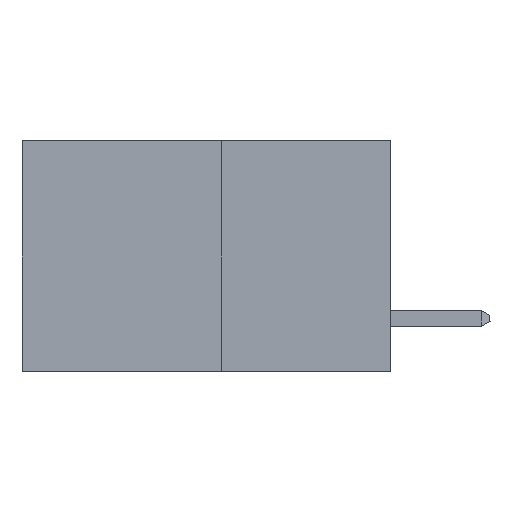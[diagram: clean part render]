
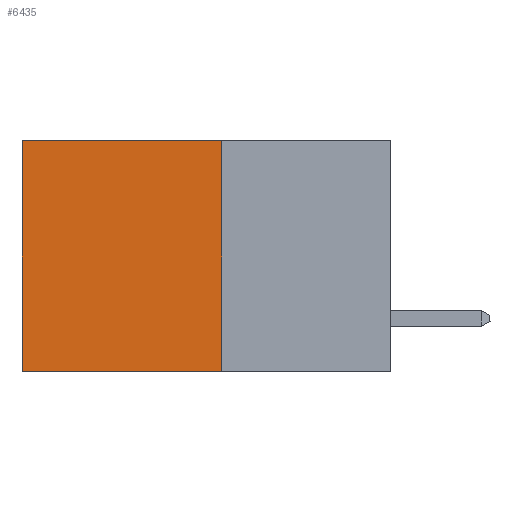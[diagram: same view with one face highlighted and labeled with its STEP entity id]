
A CAD part, left-side view. The second image highlights one B-rep face of the part: STEP entity #6435.
In plain terms, the highlighted planar face has unit normal (-1, 0, 0).
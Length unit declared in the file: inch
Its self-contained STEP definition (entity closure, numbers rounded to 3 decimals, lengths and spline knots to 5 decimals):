
#785 = VERTEX_POINT ( 'NONE', #7321 ) ;
#1035 = DIRECTION ( 'NONE',  ( 0., 0., -1. ) ) ;
#2072 = VECTOR ( 'NONE', #4828, 39.37008 ) ;
#3062 = DIRECTION ( 'NONE',  ( 0., 0., -1. ) ) ;
#3618 = CARTESIAN_POINT ( 'NONE',  ( 0.277, 0.59, -0.37 ) ) ;
#4387 = CARTESIAN_POINT ( 'NONE',  ( 0.277, 0.27, 0. ) ) ;
#4828 = DIRECTION ( 'NONE',  ( 0., 0., -1. ) ) ;
#4956 = VECTOR ( 'NONE', #12111, 39.37008 ) ;
#5126 = CARTESIAN_POINT ( 'NONE',  ( 0.277, 0.27, 0. ) ) ;
#5368 = VECTOR ( 'NONE', #13273, 39.37008 ) ;
#5540 = ORIENTED_EDGE ( 'NONE', *, *, #6653, .T. ) ;
#5718 = VERTEX_POINT ( 'NONE', #5126 ) ;
#5897 = ORIENTED_EDGE ( 'NONE', *, *, #10549, .F. ) ;
#5956 = ORIENTED_EDGE ( 'NONE', *, *, #11150, .F. ) ;
#5995 = ORIENTED_EDGE ( 'NONE', *, *, #8294, .T. ) ;
#6435 = ADVANCED_FACE ( 'NONE', ( #13445 ), #11102, .F. ) ;
#6440 = CARTESIAN_POINT ( 'NONE',  ( 0.277, 0.59, 0. ) ) ;
#6594 = VERTEX_POINT ( 'NONE', #3618 ) ;
#6653 = EDGE_CURVE ( 'NONE', #8173, #6594, #10682, .T. ) ;
#6681 = CARTESIAN_POINT ( 'NONE',  ( 0.277, 0.27, -0.37 ) ) ;
#7321 = CARTESIAN_POINT ( 'NONE',  ( 0.277, 0.27, -0.37 ) ) ;
#7776 = DIRECTION ( 'NONE',  ( 1., 0., 0. ) ) ;
#8100 = CARTESIAN_POINT ( 'NONE',  ( 0.277, 0.59, -0.37 ) ) ;
#8173 = VERTEX_POINT ( 'NONE', #6440 ) ;
#8294 = EDGE_CURVE ( 'NONE', #5718, #8173, #8655, .T. ) ;
#8655 = LINE ( 'NONE', #4387, #5368 ) ;
#8756 = CARTESIAN_POINT ( 'NONE',  ( 0.277, 0.27, -0.37 ) ) ;
#9749 = CARTESIAN_POINT ( 'NONE',  ( 0.277, 0.27, -0.37 ) ) ;
#10447 = LINE ( 'NONE', #9749, #13721 ) ;
#10549 = EDGE_CURVE ( 'NONE', #785, #6594, #13121, .T. ) ;
#10682 = LINE ( 'NONE', #8100, #2072 ) ;
#11102 = PLANE ( 'NONE',  #12303 ) ;
#11150 = EDGE_CURVE ( 'NONE', #5718, #785, #10447, .T. ) ;
#12111 = DIRECTION ( 'NONE',  ( 0., 1., 0. ) ) ;
#12303 = AXIS2_PLACEMENT_3D ( 'NONE', #6681, #7776, #1035 ) ;
#13121 = LINE ( 'NONE', #8756, #4956 ) ;
#13273 = DIRECTION ( 'NONE',  ( 0., 1., 0. ) ) ;
#13445 = FACE_OUTER_BOUND ( 'NONE', #14449, .T. ) ;
#13721 = VECTOR ( 'NONE', #3062, 39.37008 ) ;
#14449 = EDGE_LOOP ( 'NONE', ( #5540, #5897, #5956, #5995 ) ) ;
